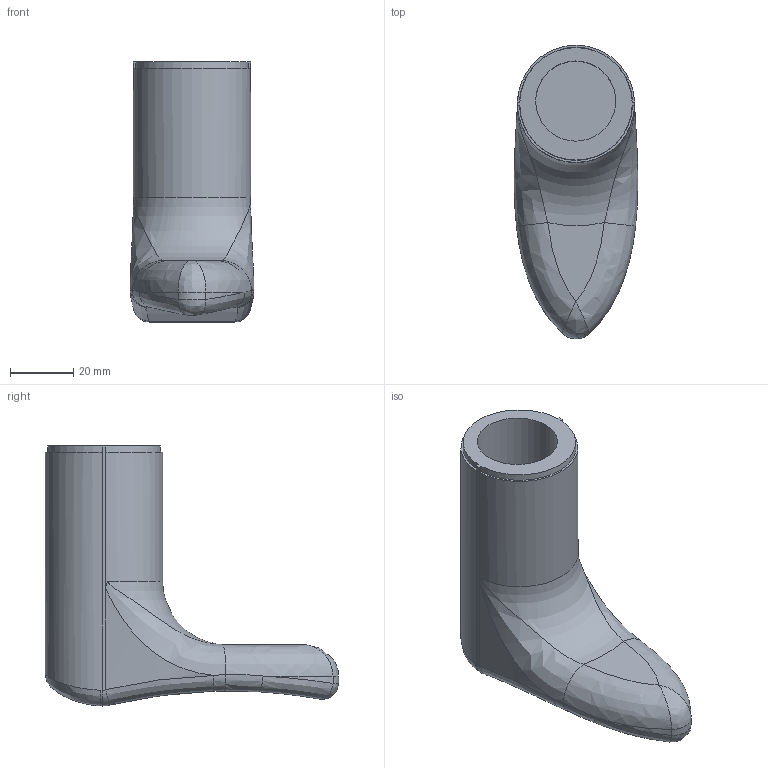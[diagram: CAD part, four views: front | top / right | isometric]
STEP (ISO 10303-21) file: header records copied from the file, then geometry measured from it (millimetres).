
FILE_DESCRIPTION (( 'STEP AP214' ), '1' );
FILE_NAME ('Hermes_v1.3.3_Stock_Rear.STEP', '2014-02-17T06:07:12', ( 'elpi' ), ( '' ), 'SwSTEP 2.0', 'SolidWorks 2013', '' );
FILE_SCHEMA (( 'AUTOMOTIVE_DESIGN' ));
Length unit declared in the file: inch
Products named in the file (1): Hermes_v1.3.3_Stock_Rear
Bounding box: 39.18 x 92.89 x 82.37 mm (x, y, z)
Volume: 85669.5 mm3; surface area: 20822.3 mm2
Topology: 1 solids, 1 shells, 44 faces, 106 edges, 64 vertices
Faces by surface type: bspline 23, plane 11, cylinder 5, torus 3, cone 2
Full cylindrical faces by diameter (mm): 25.4 x1
Entity records: 3280 total; most frequent: CARTESIAN_POINT 2387, ORIENTED_EDGE 206, DIRECTION 130, EDGE_CURVE 103, VERTEX_POINT 63, AXIS2_PLACEMENT_3D 49, EDGE_LOOP 46, FACE_OUTER_BOUND 45
